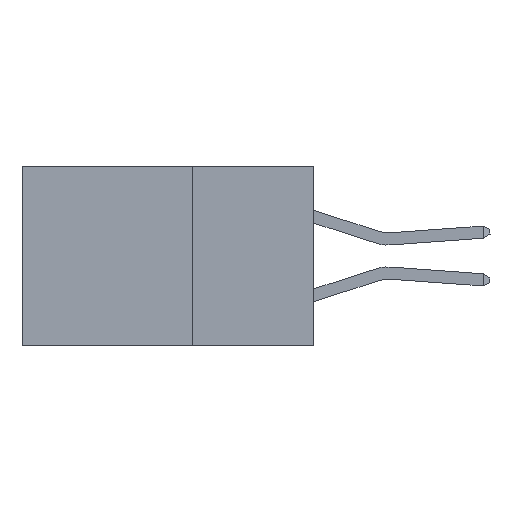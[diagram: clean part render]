
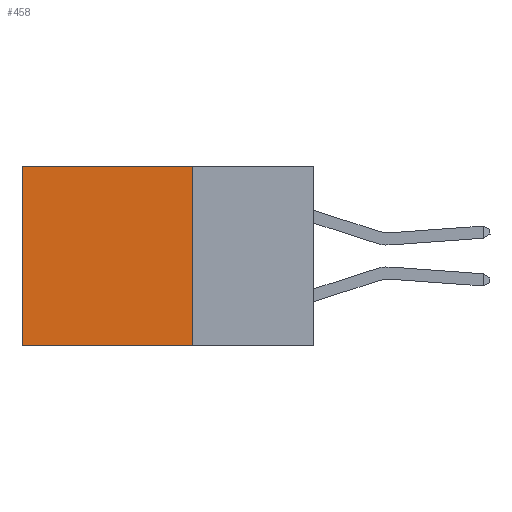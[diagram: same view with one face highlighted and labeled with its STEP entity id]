
A CAD part, left-side view. The second image highlights one B-rep face of the part: STEP entity #458.
In plain terms, the highlighted planar face has unit normal (-1, 0, 0).
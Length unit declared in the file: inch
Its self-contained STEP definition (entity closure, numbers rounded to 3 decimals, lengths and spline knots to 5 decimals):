
#458 = ADVANCED_FACE ( 'NONE', ( #16190 ), #9568, .F. ) ;
#1482 = AXIS2_PLACEMENT_3D ( 'NONE', #14862, #2939, #8254 ) ;
#1921 = CARTESIAN_POINT ( 'NONE',  ( 0.2875, 0.25, -0.37 ) ) ;
#2939 = DIRECTION ( 'NONE',  ( 1., 0., 0. ) ) ;
#3614 = DIRECTION ( 'NONE',  ( 0., 0., -1. ) ) ;
#6207 = EDGE_CURVE ( 'NONE', #14045, #11844, #16520, .T. ) ;
#6566 = CARTESIAN_POINT ( 'NONE',  ( 0.2875, 0.6, 0. ) ) ;
#6638 = DIRECTION ( 'NONE',  ( 0., 1., 0. ) ) ;
#8017 = ORIENTED_EDGE ( 'NONE', *, *, #15074, .T. ) ;
#8254 = DIRECTION ( 'NONE',  ( 0., 0., -1. ) ) ;
#9568 = PLANE ( 'NONE',  #1482 ) ;
#9608 = LINE ( 'NONE', #14553, #12545 ) ;
#9738 = LINE ( 'NONE', #13462, #17028 ) ;
#11100 = CARTESIAN_POINT ( 'NONE',  ( 0.2875, 0.25, -0.37 ) ) ;
#11109 = ORIENTED_EDGE ( 'NONE', *, *, #15642, .T. ) ;
#11164 = CARTESIAN_POINT ( 'NONE',  ( 0.2875, 0.25, 0. ) ) ;
#11844 = VERTEX_POINT ( 'NONE', #13823 ) ;
#12150 = ORIENTED_EDGE ( 'NONE', *, *, #6207, .F. ) ;
#12238 = VERTEX_POINT ( 'NONE', #15603 ) ;
#12545 = VECTOR ( 'NONE', #6638, 39.37008 ) ;
#13462 = CARTESIAN_POINT ( 'NONE',  ( 0.2875, 0.25, 0. ) ) ;
#13605 = ORIENTED_EDGE ( 'NONE', *, *, #14789, .F. ) ;
#13823 = CARTESIAN_POINT ( 'NONE',  ( 0.2875, 0.6, -0.37 ) ) ;
#13966 = VERTEX_POINT ( 'NONE', #11164 ) ;
#14045 = VERTEX_POINT ( 'NONE', #1921 ) ;
#14550 = EDGE_LOOP ( 'NONE', ( #8017, #12150, #13605, #11109 ) ) ;
#14553 = CARTESIAN_POINT ( 'NONE',  ( 0.2875, 0.25, 0. ) ) ;
#14789 = EDGE_CURVE ( 'NONE', #13966, #14045, #9738, .T. ) ;
#14820 = VECTOR ( 'NONE', #15587, 39.37008 ) ;
#14862 = CARTESIAN_POINT ( 'NONE',  ( 0.2875, 0.25, 0. ) ) ;
#15068 = VECTOR ( 'NONE', #3614, 39.37008 ) ;
#15074 = EDGE_CURVE ( 'NONE', #12238, #11844, #17216, .T. ) ;
#15587 = DIRECTION ( 'NONE',  ( 0., 1., 0. ) ) ;
#15603 = CARTESIAN_POINT ( 'NONE',  ( 0.2875, 0.6, 0. ) ) ;
#15642 = EDGE_CURVE ( 'NONE', #13966, #12238, #9608, .T. ) ;
#16182 = DIRECTION ( 'NONE',  ( 0., 0., -1. ) ) ;
#16190 = FACE_OUTER_BOUND ( 'NONE', #14550, .T. ) ;
#16520 = LINE ( 'NONE', #11100, #14820 ) ;
#17028 = VECTOR ( 'NONE', #16182, 39.37008 ) ;
#17216 = LINE ( 'NONE', #6566, #15068 ) ;
